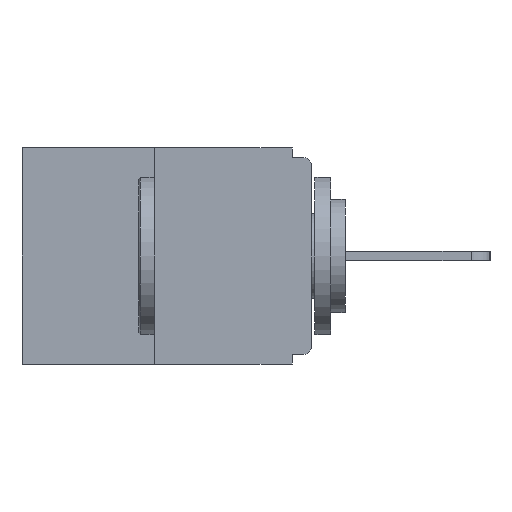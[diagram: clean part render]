
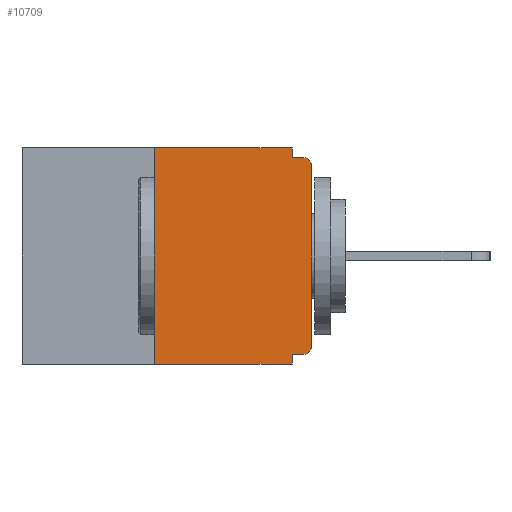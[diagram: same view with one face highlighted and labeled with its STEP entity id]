
A CAD part, left-side view. The second image highlights one B-rep face of the part: STEP entity #10709.
In plain terms, the highlighted planar face has unit normal (-1, 0, 0).
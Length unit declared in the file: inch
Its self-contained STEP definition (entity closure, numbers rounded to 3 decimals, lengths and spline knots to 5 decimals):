
#153 = CARTESIAN_POINT ( 'NONE',  ( 0., 0., -0.03 ) ) ;
#211 = DIRECTION ( 'NONE',  ( 0., 0., -1. ) ) ;
#331 = CARTESIAN_POINT ( 'NONE',  ( 0., 0.031, -0.343 ) ) ;
#820 = CARTESIAN_POINT ( 'NONE',  ( 0., 0.015, -0.03 ) ) ;
#864 = CARTESIAN_POINT ( 'NONE',  ( 0., 0.031, -0.015 ) ) ;
#1762 = CARTESIAN_POINT ( 'NONE',  ( 0., 0.031, -0.343 ) ) ;
#2121 = DIRECTION ( 'NONE',  ( -1., 0., 0. ) ) ;
#2141 = DIRECTION ( 'NONE',  ( 0., -1., 0. ) ) ;
#3270 = EDGE_CURVE ( 'NONE', #14389, #7019, #9916, .T. ) ;
#3504 = VECTOR ( 'NONE', #211, 39.37008 ) ;
#3827 = EDGE_CURVE ( 'NONE', #8040, #5000, #7739, .T. ) ;
#3954 = CARTESIAN_POINT ( 'NONE',  ( 0., 0., -0.015 ) ) ;
#3962 = EDGE_CURVE ( 'NONE', #7019, #5000, #18531, .T. ) ;
#4251 = CIRCLE ( 'NONE', #12887, 0.015 ) ;
#4445 = VECTOR ( 'NONE', #12936, 39.37008 ) ;
#4450 = ORIENTED_EDGE ( 'NONE', *, *, #6419, .F. ) ;
#4510 = ORIENTED_EDGE ( 'NONE', *, *, #3962, .T. ) ;
#4552 = ORIENTED_EDGE ( 'NONE', *, *, #18267, .T. ) ;
#4903 = ORIENTED_EDGE ( 'NONE', *, *, #8051, .F. ) ;
#4950 = EDGE_CURVE ( 'NONE', #14481, #13395, #17920, .T. ) ;
#5000 = VERTEX_POINT ( 'NONE', #8125 ) ;
#5389 = CARTESIAN_POINT ( 'NONE',  ( 0., 0.46, 0. ) ) ;
#5569 = CARTESIAN_POINT ( 'NONE',  ( 0., 0.46, 0. ) ) ;
#5674 = CARTESIAN_POINT ( 'NONE',  ( 0., 0.25, 0. ) ) ;
#6080 = CARTESIAN_POINT ( 'NONE',  ( 0., 0.25, 0. ) ) ;
#6108 = CARTESIAN_POINT ( 'NONE',  ( 0., 0.031, 0. ) ) ;
#6118 = AXIS2_PLACEMENT_3D ( 'NONE', #5389, #20484, #10505 ) ;
#6419 = EDGE_CURVE ( 'NONE', #17299, #14086, #19642, .T. ) ;
#6771 = CARTESIAN_POINT ( 'NONE',  ( 0., 0.031, 0. ) ) ;
#6946 = DIRECTION ( 'NONE',  ( 0., 1., 0. ) ) ;
#7019 = VERTEX_POINT ( 'NONE', #153 ) ;
#7253 = LINE ( 'NONE', #12780, #20118 ) ;
#7716 = CARTESIAN_POINT ( 'NONE',  ( 0., 0.015, -0.328 ) ) ;
#7739 = LINE ( 'NONE', #3954, #11721 ) ;
#7924 = FACE_OUTER_BOUND ( 'NONE', #9708, .T. ) ;
#8040 = VERTEX_POINT ( 'NONE', #864 ) ;
#8051 = EDGE_CURVE ( 'NONE', #14086, #15238, #21381, .T. ) ;
#8125 = CARTESIAN_POINT ( 'NONE',  ( 0., 0.015, -0.015 ) ) ;
#8403 = VECTOR ( 'NONE', #2141, 39.37008 ) ;
#8797 = PLANE ( 'NONE',  #6118 ) ;
#8976 = ORIENTED_EDGE ( 'NONE', *, *, #11870, .F. ) ;
#9708 = EDGE_LOOP ( 'NONE', ( #16706, #19576, #12586, #4903, #4450, #4552, #18758, #4510, #10512, #8976 ) ) ;
#9916 = LINE ( 'NONE', #11279, #14415 ) ;
#10505 = DIRECTION ( 'NONE',  ( 0., 0., -1. ) ) ;
#10512 = ORIENTED_EDGE ( 'NONE', *, *, #3827, .F. ) ;
#10709 = ADVANCED_FACE ( 'NONE', ( #7924 ), #8797, .F. ) ;
#11254 = DIRECTION ( 'NONE',  ( 0., 0., 1. ) ) ;
#11279 = CARTESIAN_POINT ( 'NONE',  ( 0., 0., 0. ) ) ;
#11387 = CARTESIAN_POINT ( 'NONE',  ( 0., 0.25, -0.343 ) ) ;
#11721 = VECTOR ( 'NONE', #15268, 39.37008 ) ;
#11870 = EDGE_CURVE ( 'NONE', #13527, #8040, #12798, .T. ) ;
#12350 = CARTESIAN_POINT ( 'NONE',  ( 0., 0.015, -0.313 ) ) ;
#12523 = AXIS2_PLACEMENT_3D ( 'NONE', #820, #20410, #21737 ) ;
#12586 = ORIENTED_EDGE ( 'NONE', *, *, #16703, .T. ) ;
#12770 = CARTESIAN_POINT ( 'NONE',  ( 0., 0., -0.313 ) ) ;
#12780 = CARTESIAN_POINT ( 'NONE',  ( 0., 0.46, -0.343 ) ) ;
#12798 = LINE ( 'NONE', #6771, #16241 ) ;
#12887 = AXIS2_PLACEMENT_3D ( 'NONE', #12350, #2121, #14072 ) ;
#12936 = DIRECTION ( 'NONE',  ( 0., 0., 1. ) ) ;
#13395 = VERTEX_POINT ( 'NONE', #5674 ) ;
#13527 = VERTEX_POINT ( 'NONE', #6108 ) ;
#13699 = CARTESIAN_POINT ( 'NONE',  ( 0., 0.031, -0.328 ) ) ;
#14072 = DIRECTION ( 'NONE',  ( 0., 0., -1. ) ) ;
#14086 = VERTEX_POINT ( 'NONE', #13699 ) ;
#14389 = VERTEX_POINT ( 'NONE', #12770 ) ;
#14415 = VECTOR ( 'NONE', #11254, 39.37008 ) ;
#14481 = VERTEX_POINT ( 'NONE', #11387 ) ;
#15238 = VERTEX_POINT ( 'NONE', #1762 ) ;
#15268 = DIRECTION ( 'NONE',  ( 0., -1., 0. ) ) ;
#15346 = EDGE_CURVE ( 'NONE', #13395, #13527, #17371, .T. ) ;
#16241 = VECTOR ( 'NONE', #20186, 39.37008 ) ;
#16470 = CARTESIAN_POINT ( 'NONE',  ( 0., 0., -0.328 ) ) ;
#16703 = EDGE_CURVE ( 'NONE', #14481, #15238, #7253, .T. ) ;
#16706 = ORIENTED_EDGE ( 'NONE', *, *, #15346, .F. ) ;
#17299 = VERTEX_POINT ( 'NONE', #7716 ) ;
#17371 = LINE ( 'NONE', #5569, #8403 ) ;
#17920 = LINE ( 'NONE', #6080, #4445 ) ;
#18267 = EDGE_CURVE ( 'NONE', #17299, #14389, #4251, .T. ) ;
#18531 = CIRCLE ( 'NONE', #12523, 0.015 ) ;
#18758 = ORIENTED_EDGE ( 'NONE', *, *, #3270, .T. ) ;
#19131 = VECTOR ( 'NONE', #6946, 39.37008 ) ;
#19495 = DIRECTION ( 'NONE',  ( 0., -1., 0. ) ) ;
#19576 = ORIENTED_EDGE ( 'NONE', *, *, #4950, .F. ) ;
#19642 = LINE ( 'NONE', #16470, #19131 ) ;
#20118 = VECTOR ( 'NONE', #19495, 39.37008 ) ;
#20186 = DIRECTION ( 'NONE',  ( 0., 0., -1. ) ) ;
#20410 = DIRECTION ( 'NONE',  ( -1., 0., 0. ) ) ;
#20484 = DIRECTION ( 'NONE',  ( 1., 0., 0. ) ) ;
#21381 = LINE ( 'NONE', #331, #3504 ) ;
#21737 = DIRECTION ( 'NONE',  ( 0., 0., -1. ) ) ;
